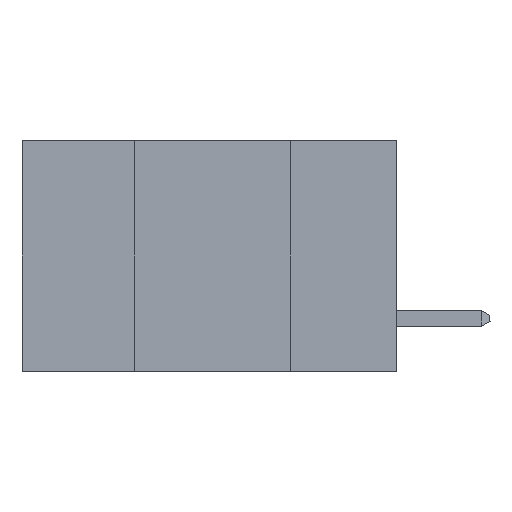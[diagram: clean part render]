
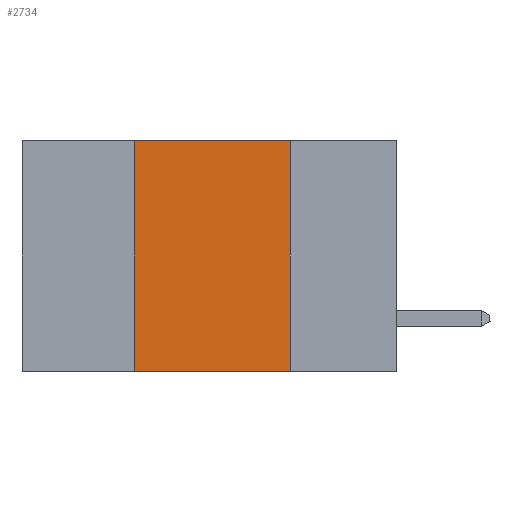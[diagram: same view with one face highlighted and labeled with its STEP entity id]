
A CAD part, left-side view. The second image highlights one B-rep face of the part: STEP entity #2734.
In plain terms, the highlighted planar face has unit normal (-1, 0, 0).
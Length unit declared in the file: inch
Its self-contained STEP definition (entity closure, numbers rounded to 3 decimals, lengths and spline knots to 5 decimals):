
#830 = CARTESIAN_POINT ( 'NONE',  ( 0., 0.6, 0. ) ) ;
#1384 = VERTEX_POINT ( 'NONE', #2406 ) ;
#2406 = CARTESIAN_POINT ( 'NONE',  ( 0., 0.17, -0.37 ) ) ;
#2638 = DIRECTION ( 'NONE',  ( 0., -1., 0. ) ) ;
#2734 = ADVANCED_FACE ( 'NONE', ( #19510 ), #27367, .F. ) ;
#3057 = EDGE_CURVE ( 'NONE', #7837, #11073, #22308, .T. ) ;
#4389 = CARTESIAN_POINT ( 'NONE',  ( 0., 0.42, -0.37 ) ) ;
#6632 = EDGE_CURVE ( 'NONE', #21984, #7837, #14346, .T. ) ;
#6828 = DIRECTION ( 'NONE',  ( 0., 0., 1. ) ) ;
#6868 = CARTESIAN_POINT ( 'NONE',  ( 0., 0.42, 0. ) ) ;
#7837 = VERTEX_POINT ( 'NONE', #26354 ) ;
#7914 = EDGE_CURVE ( 'NONE', #11073, #1384, #22104, .T. ) ;
#11073 = VERTEX_POINT ( 'NONE', #15640 ) ;
#11241 = CARTESIAN_POINT ( 'NONE',  ( 0., 0.6, 0. ) ) ;
#12005 = AXIS2_PLACEMENT_3D ( 'NONE', #11241, #28741, #28435 ) ;
#12211 = VECTOR ( 'NONE', #24423, 39.37008 ) ;
#14129 = CARTESIAN_POINT ( 'NONE',  ( 0., 0.6, -0.37 ) ) ;
#14346 = LINE ( 'NONE', #6868, #24924 ) ;
#14611 = VECTOR ( 'NONE', #2638, 39.37008 ) ;
#15444 = CARTESIAN_POINT ( 'NONE',  ( 0., 0.17, 0. ) ) ;
#15640 = CARTESIAN_POINT ( 'NONE',  ( 0., 0.17, 0. ) ) ;
#16052 = EDGE_LOOP ( 'NONE', ( #24913, #18992, #26671, #21475 ) ) ;
#18992 = ORIENTED_EDGE ( 'NONE', *, *, #3057, .F. ) ;
#19510 = FACE_OUTER_BOUND ( 'NONE', #16052, .T. ) ;
#20403 = EDGE_CURVE ( 'NONE', #21984, #1384, #22068, .T. ) ;
#20466 = DIRECTION ( 'NONE',  ( 0., -1., 0. ) ) ;
#21475 = ORIENTED_EDGE ( 'NONE', *, *, #20403, .T. ) ;
#21984 = VERTEX_POINT ( 'NONE', #4389 ) ;
#22068 = LINE ( 'NONE', #14129, #14611 ) ;
#22104 = LINE ( 'NONE', #15444, #12211 ) ;
#22308 = LINE ( 'NONE', #830, #27513 ) ;
#24423 = DIRECTION ( 'NONE',  ( 0., 0., -1. ) ) ;
#24913 = ORIENTED_EDGE ( 'NONE', *, *, #7914, .F. ) ;
#24924 = VECTOR ( 'NONE', #6828, 39.37008 ) ;
#26354 = CARTESIAN_POINT ( 'NONE',  ( 0., 0.42, 0. ) ) ;
#26671 = ORIENTED_EDGE ( 'NONE', *, *, #6632, .F. ) ;
#27367 = PLANE ( 'NONE',  #12005 ) ;
#27513 = VECTOR ( 'NONE', #20466, 39.37008 ) ;
#28435 = DIRECTION ( 'NONE',  ( 0., 0., -1. ) ) ;
#28741 = DIRECTION ( 'NONE',  ( 1., 0., 0. ) ) ;
